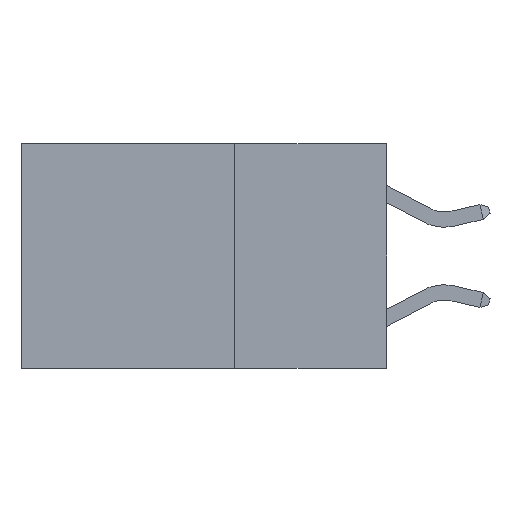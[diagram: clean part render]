
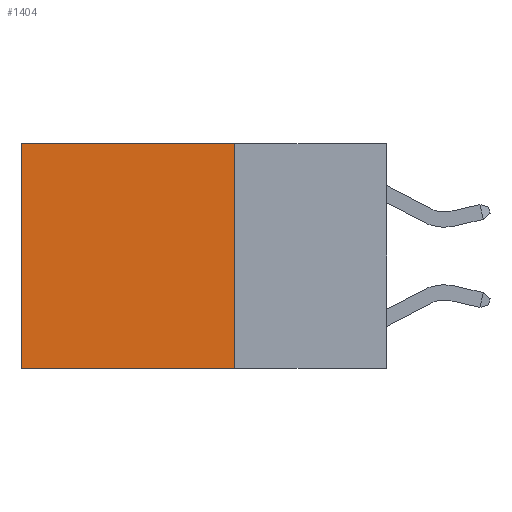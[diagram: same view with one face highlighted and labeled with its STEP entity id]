
A CAD part, left-side view. The second image highlights one B-rep face of the part: STEP entity #1404.
In plain terms, the highlighted planar face has unit normal (-1, 0, 0).
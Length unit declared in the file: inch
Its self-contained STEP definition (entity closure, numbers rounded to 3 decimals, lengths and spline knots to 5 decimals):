
#344 = CARTESIAN_POINT ( 'NONE',  ( 0.2625, 0.25, 0. ) ) ;
#526 = EDGE_CURVE ( 'NONE', #12042, #2477, #14526, .T. ) ;
#1404 = ADVANCED_FACE ( 'NONE', ( #9747 ), #11500, .F. ) ;
#1640 = CARTESIAN_POINT ( 'NONE',  ( 0.2625, 0.25, 0. ) ) ;
#1802 = CARTESIAN_POINT ( 'NONE',  ( 0.2625, 0.25, 0. ) ) ;
#1848 = DIRECTION ( 'NONE',  ( 0., 0., -1. ) ) ;
#2477 = VERTEX_POINT ( 'NONE', #14966 ) ;
#3162 = EDGE_CURVE ( 'NONE', #17542, #2477, #17184, .T. ) ;
#3664 = EDGE_CURVE ( 'NONE', #9136, #17542, #15741, .T. ) ;
#4210 = ORIENTED_EDGE ( 'NONE', *, *, #526, .T. ) ;
#5578 = DIRECTION ( 'NONE',  ( 0., 0., -1. ) ) ;
#7228 = AXIS2_PLACEMENT_3D ( 'NONE', #14354, #19327, #1848 ) ;
#8052 = LINE ( 'NONE', #344, #9775 ) ;
#8632 = CARTESIAN_POINT ( 'NONE',  ( 0.2625, 0.6, 0. ) ) ;
#9136 = VERTEX_POINT ( 'NONE', #1640 ) ;
#9250 = ORIENTED_EDGE ( 'NONE', *, *, #3162, .F. ) ;
#9747 = FACE_OUTER_BOUND ( 'NONE', #11817, .T. ) ;
#9775 = VECTOR ( 'NONE', #14931, 39.37008 ) ;
#9912 = DIRECTION ( 'NONE',  ( 0., 0., -1. ) ) ;
#11277 = DIRECTION ( 'NONE',  ( 0., 1., 0. ) ) ;
#11500 = PLANE ( 'NONE',  #7228 ) ;
#11817 = EDGE_LOOP ( 'NONE', ( #4210, #9250, #14047, #13909 ) ) ;
#11926 = EDGE_CURVE ( 'NONE', #9136, #12042, #8052, .T. ) ;
#12042 = VERTEX_POINT ( 'NONE', #16176 ) ;
#13026 = CARTESIAN_POINT ( 'NONE',  ( 0.2625, 0.25, -0.37 ) ) ;
#13909 = ORIENTED_EDGE ( 'NONE', *, *, #11926, .T. ) ;
#14047 = ORIENTED_EDGE ( 'NONE', *, *, #3664, .F. ) ;
#14354 = CARTESIAN_POINT ( 'NONE',  ( 0.2625, 0.25, 0. ) ) ;
#14526 = LINE ( 'NONE', #8632, #16042 ) ;
#14738 = VECTOR ( 'NONE', #9912, 39.37008 ) ;
#14931 = DIRECTION ( 'NONE',  ( 0., 1., 0. ) ) ;
#14966 = CARTESIAN_POINT ( 'NONE',  ( 0.2625, 0.6, -0.37 ) ) ;
#15741 = LINE ( 'NONE', #1802, #14738 ) ;
#16042 = VECTOR ( 'NONE', #5578, 39.37008 ) ;
#16176 = CARTESIAN_POINT ( 'NONE',  ( 0.2625, 0.6, 0. ) ) ;
#17184 = LINE ( 'NONE', #17283, #17450 ) ;
#17283 = CARTESIAN_POINT ( 'NONE',  ( 0.2625, 0.25, -0.37 ) ) ;
#17450 = VECTOR ( 'NONE', #11277, 39.37008 ) ;
#17542 = VERTEX_POINT ( 'NONE', #13026 ) ;
#19327 = DIRECTION ( 'NONE',  ( 1., 0., 0. ) ) ;
